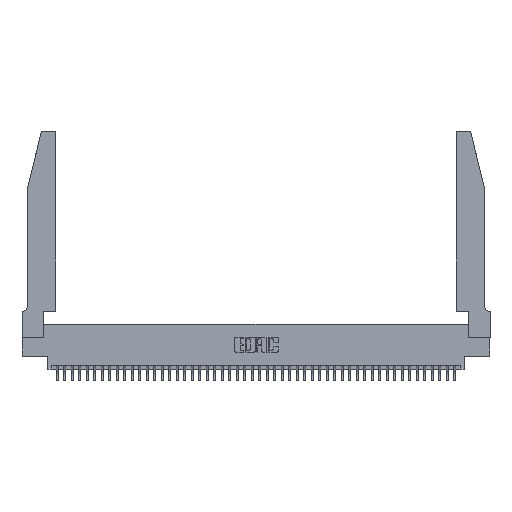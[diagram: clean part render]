
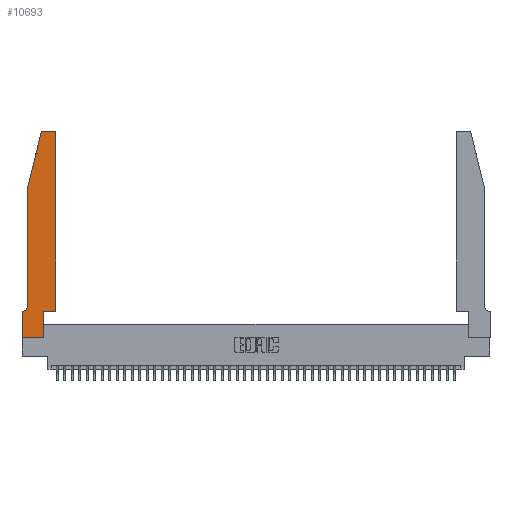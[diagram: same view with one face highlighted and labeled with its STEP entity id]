
A CAD part, top view. The second image highlights one B-rep face of the part: STEP entity #10693.
In plain terms, the highlighted planar face has unit normal (0, 0, 1).
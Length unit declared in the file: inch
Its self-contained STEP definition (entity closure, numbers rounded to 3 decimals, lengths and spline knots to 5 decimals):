
#803 = VECTOR ( 'NONE', #18502, 39.37008 ) ;
#943 = CARTESIAN_POINT ( 'NONE',  ( 0.0755, 0.35, 0.37 ) ) ;
#1629 = EDGE_CURVE ( 'NONE', #18018, #7223, #11248, .T. ) ;
#1849 = VECTOR ( 'NONE', #24862, 39.37008 ) ;
#2707 = AXIS2_PLACEMENT_3D ( 'NONE', #31563, #28003, #35131 ) ;
#4505 = DIRECTION ( 'NONE',  ( -1., 0., 0. ) ) ;
#5180 = ORIENTED_EDGE ( 'NONE', *, *, #21810, .T. ) ;
#5219 = EDGE_CURVE ( 'NONE', #35134, #34744, #36720, .T. ) ;
#5708 = CARTESIAN_POINT ( 'NONE',  ( 0.4505, 0.35, 0.37 ) ) ;
#6887 = CARTESIAN_POINT ( 'NONE',  ( 0.2865, 0.35, 0.37 ) ) ;
#7223 = VERTEX_POINT ( 'NONE', #15018 ) ;
#7362 = VERTEX_POINT ( 'NONE', #26216 ) ;
#7590 = VERTEX_POINT ( 'NONE', #5708 ) ;
#7991 = LINE ( 'NONE', #40222, #32398 ) ;
#8275 = EDGE_CURVE ( 'NONE', #36696, #35134, #14170, .T. ) ;
#9078 = ORIENTED_EDGE ( 'NONE', *, *, #35441, .T. ) ;
#10384 = ORIENTED_EDGE ( 'NONE', *, *, #28385, .T. ) ;
#10693 = ADVANCED_FACE ( 'NONE', ( #20508 ), #35204, .T. ) ;
#11248 = LINE ( 'NONE', #6887, #1849 ) ;
#13910 = DIRECTION ( 'NONE',  ( 1., 0., 0. ) ) ;
#14069 = LINE ( 'NONE', #40395, #803 ) ;
#14170 = LINE ( 'NONE', #27838, #15879 ) ;
#14738 = CARTESIAN_POINT ( 'NONE',  ( 0., 0., 0.37 ) ) ;
#15018 = CARTESIAN_POINT ( 'NONE',  ( 0.2865, 0.35, 0.37 ) ) ;
#15169 = DIRECTION ( 'NONE',  ( 0., 0., -1. ) ) ;
#15513 = CARTESIAN_POINT ( 'NONE',  ( 0.0755, 0.42, 0.37 ) ) ;
#15810 = DIRECTION ( 'NONE',  ( 1., 0., 0. ) ) ;
#15879 = VECTOR ( 'NONE', #31242, 39.37008 ) ;
#16265 = CARTESIAN_POINT ( 'NONE',  ( 0.4205, 2.72, 0.37 ) ) ;
#16506 = CARTESIAN_POINT ( 'NONE',  ( 0.0755, 2., 0.37 ) ) ;
#17080 = VECTOR ( 'NONE', #40518, 39.37008 ) ;
#17171 = EDGE_LOOP ( 'NONE', ( #10384, #31993, #42633, #32666, #24694, #17299, #40520, #28211, #25247, #9078, #5180, #17460 ) ) ;
#17299 = ORIENTED_EDGE ( 'NONE', *, *, #32461, .T. ) ;
#17310 = VECTOR ( 'NONE', #43258, 39.37008 ) ;
#17389 = CIRCLE ( 'NONE', #19268, 0.03 ) ;
#17460 = ORIENTED_EDGE ( 'NONE', *, *, #42408, .T. ) ;
#18018 = VERTEX_POINT ( 'NONE', #27367 ) ;
#18502 = DIRECTION ( 'NONE',  ( 0., 1., 0. ) ) ;
#19268 = AXIS2_PLACEMENT_3D ( 'NONE', #16265, #41101, #15810 ) ;
#20508 = FACE_OUTER_BOUND ( 'NONE', #17171, .T. ) ;
#20936 = EDGE_CURVE ( 'NONE', #43766, #36696, #32503, .T. ) ;
#21295 = CARTESIAN_POINT ( 'NONE',  ( 0., 0.35, 0.37 ) ) ;
#21568 = CIRCLE ( 'NONE', #2707, 0.03 ) ;
#21810 = EDGE_CURVE ( 'NONE', #7590, #7362, #14069, .T. ) ;
#23350 = AXIS2_PLACEMENT_3D ( 'NONE', #32550, #15169, #29303 ) ;
#24694 = ORIENTED_EDGE ( 'NONE', *, *, #5219, .T. ) ;
#24862 = DIRECTION ( 'NONE',  ( 0., 1., 0. ) ) ;
#25247 = ORIENTED_EDGE ( 'NONE', *, *, #1629, .T. ) ;
#25852 = VECTOR ( 'NONE', #13910, 39.37008 ) ;
#25917 = VERTEX_POINT ( 'NONE', #34337 ) ;
#26216 = CARTESIAN_POINT ( 'NONE',  ( 0.4505, 2.72, 0.37 ) ) ;
#26377 = EDGE_CURVE ( 'NONE', #43155, #45259, #32626, .T. ) ;
#27357 = LINE ( 'NONE', #36311, #17310 ) ;
#27367 = CARTESIAN_POINT ( 'NONE',  ( 0.2865, 0., 0.37 ) ) ;
#27838 = CARTESIAN_POINT ( 'NONE',  ( 0.0755, 2., 0.37 ) ) ;
#28003 = DIRECTION ( 'NONE',  ( 0., 0., 1. ) ) ;
#28211 = ORIENTED_EDGE ( 'NONE', *, *, #44102, .T. ) ;
#28385 = EDGE_CURVE ( 'NONE', #35600, #25917, #7991, .T. ) ;
#29163 = LINE ( 'NONE', #38306, #25852 ) ;
#29303 = DIRECTION ( 'NONE',  ( -1., 0., 0. ) ) ;
#31242 = DIRECTION ( 'NONE',  ( 0., -1., 0. ) ) ;
#31486 = CARTESIAN_POINT ( 'NONE',  ( 0., 0.35, 0.37 ) ) ;
#31563 = CARTESIAN_POINT ( 'NONE',  ( 0.284, 2.72, 0.37 ) ) ;
#31993 = ORIENTED_EDGE ( 'NONE', *, *, #45744, .T. ) ;
#32398 = VECTOR ( 'NONE', #39917, 39.37008 ) ;
#32461 = EDGE_CURVE ( 'NONE', #34744, #43155, #38296, .T. ) ;
#32503 = LINE ( 'NONE', #39534, #33053 ) ;
#32550 = CARTESIAN_POINT ( 'NONE',  ( 0.0055, 0.42, 0.37 ) ) ;
#32626 = LINE ( 'NONE', #14738, #17080 ) ;
#32666 = ORIENTED_EDGE ( 'NONE', *, *, #8275, .T. ) ;
#33053 = VECTOR ( 'NONE', #35640, 39.37008 ) ;
#33876 = CARTESIAN_POINT ( 'NONE',  ( 0.0055, 0.35, 0.37 ) ) ;
#34337 = CARTESIAN_POINT ( 'NONE',  ( 0.284, 2.75, 0.37 ) ) ;
#34414 = VECTOR ( 'NONE', #4505, 39.37008 ) ;
#34603 = DIRECTION ( 'NONE',  ( 0., 0., 1. ) ) ;
#34744 = VERTEX_POINT ( 'NONE', #33876 ) ;
#35131 = DIRECTION ( 'NONE',  ( 1., 0., 0. ) ) ;
#35134 = VERTEX_POINT ( 'NONE', #15513 ) ;
#35204 = PLANE ( 'NONE',  #38640 ) ;
#35441 = EDGE_CURVE ( 'NONE', #7223, #7590, #29163, .T. ) ;
#35600 = VERTEX_POINT ( 'NONE', #35632 ) ;
#35632 = CARTESIAN_POINT ( 'NONE',  ( 0.4205, 2.75, 0.37 ) ) ;
#35640 = DIRECTION ( 'NONE',  ( -0.239, -0.971, 0. ) ) ;
#36311 = CARTESIAN_POINT ( 'NONE',  ( 0., 0., 0.37 ) ) ;
#36696 = VERTEX_POINT ( 'NONE', #16506 ) ;
#36720 = CIRCLE ( 'NONE', #23350, 0.07 ) ;
#38189 = DIRECTION ( 'NONE',  ( 1., 0., 0. ) ) ;
#38296 = LINE ( 'NONE', #943, #34414 ) ;
#38306 = CARTESIAN_POINT ( 'NONE',  ( 0.4505, 0.35, 0.37 ) ) ;
#38640 = AXIS2_PLACEMENT_3D ( 'NONE', #31486, #34603, #38189 ) ;
#39534 = CARTESIAN_POINT ( 'NONE',  ( 0.0755, 2., 0.37 ) ) ;
#39917 = DIRECTION ( 'NONE',  ( -1., 0., 0. ) ) ;
#40185 = CARTESIAN_POINT ( 'NONE',  ( 0., 0., 0.37 ) ) ;
#40222 = CARTESIAN_POINT ( 'NONE',  ( 0.2605, 2.75, 0.37 ) ) ;
#40395 = CARTESIAN_POINT ( 'NONE',  ( 0.4505, 0.35, 0.37 ) ) ;
#40518 = DIRECTION ( 'NONE',  ( 0., -1., 0. ) ) ;
#40520 = ORIENTED_EDGE ( 'NONE', *, *, #26377, .T. ) ;
#41101 = DIRECTION ( 'NONE',  ( 0., 0., 1. ) ) ;
#42408 = EDGE_CURVE ( 'NONE', #7362, #35600, #17389, .T. ) ;
#42633 = ORIENTED_EDGE ( 'NONE', *, *, #20936, .T. ) ;
#43155 = VERTEX_POINT ( 'NONE', #21295 ) ;
#43258 = DIRECTION ( 'NONE',  ( 1., 0., 0. ) ) ;
#43766 = VERTEX_POINT ( 'NONE', #44957 ) ;
#44102 = EDGE_CURVE ( 'NONE', #45259, #18018, #27357, .T. ) ;
#44957 = CARTESIAN_POINT ( 'NONE',  ( 0.25487, 2.72718, 0.37 ) ) ;
#45259 = VERTEX_POINT ( 'NONE', #40185 ) ;
#45744 = EDGE_CURVE ( 'NONE', #25917, #43766, #21568, .T. ) ;
